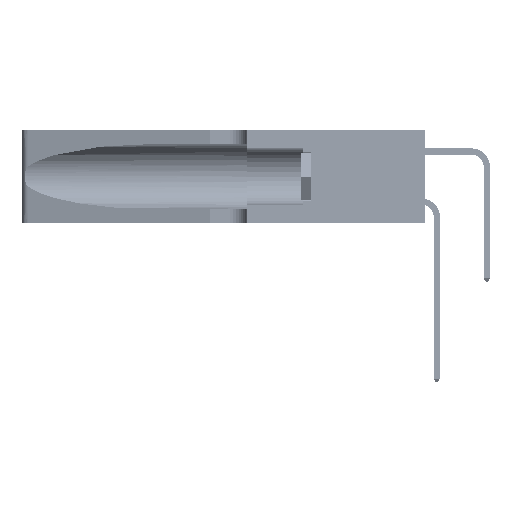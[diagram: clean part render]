
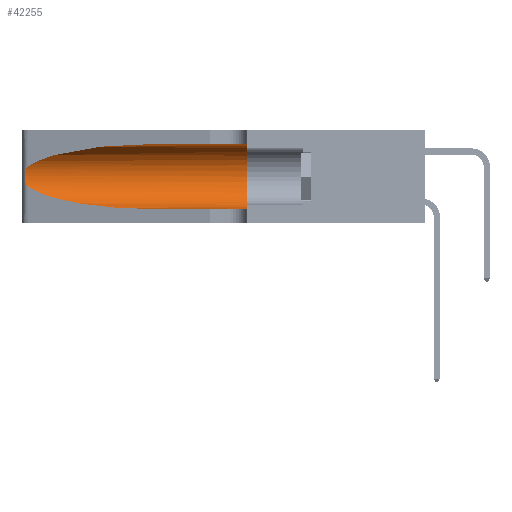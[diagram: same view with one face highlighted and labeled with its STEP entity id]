
A CAD part, left-side view. The second image highlights one B-rep face of the part: STEP entity #42255.
In plain terms, the highlighted cylindrical face has radius 3.308 mm (diameter 6.617 mm), a partial arc.
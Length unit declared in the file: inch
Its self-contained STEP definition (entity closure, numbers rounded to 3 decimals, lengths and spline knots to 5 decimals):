
#624 = VECTOR ( 'NONE', #36243, 39.37008 ) ;
#785 = VERTEX_POINT ( 'NONE', #15672 ) ;
#1450 = CARTESIAN_POINT ( 'NONE',  ( 0.1305, 0.35, 0.05475 ) ) ;
#1660 = ORIENTED_EDGE ( 'NONE', *, *, #38935, .F. ) ;
#1837 = LINE ( 'NONE', #47042, #624 ) ;
#1852 = VERTEX_POINT ( 'NONE', #19064 ) ;
#2015 = CARTESIAN_POINT ( 'NONE',  ( 0.25555, 1.22994, 0.2215 ) ) ;
#2172 = CARTESIAN_POINT ( 'NONE',  ( 0.26018, 1.23835, 0.19895 ) ) ;
#2645 = CIRCLE ( 'NONE', #7533, 0.13025 ) ;
#3365 = VECTOR ( 'NONE', #14960, 39.37008 ) ;
#3502 = EDGE_CURVE ( 'NONE', #17841, #41632, #1837, .T. ) ;
#3715 = CARTESIAN_POINT ( 'NONE',  ( 0.1305, 0.72297, 0.05475 ) ) ;
#5640 = CARTESIAN_POINT ( 'NONE',  ( 0.1305, 0.35, 0.185 ) ) ;
#5896 = CARTESIAN_POINT ( 'NONE',  ( 0.26075, 1.23896, 0.178 ) ) ;
#6258 = EDGE_CURVE ( 'NONE', #11419, #1852, #12007, .T. ) ;
#6636 =( BOUNDED_CURVE ( )  B_SPLINE_CURVE ( 3, ( #35171, #35021, #38819, #17061 ),
 .UNSPECIFIED., .F., .F. ) 
 B_SPLINE_CURVE_WITH_KNOTS ( ( 4, 4 ),
 ( 1.5708, 2.84003 ),
 .UNSPECIFIED. ) 
 CURVE ( )  GEOMETRIC_REPRESENTATION_ITEM ( )  RATIONAL_B_SPLINE_CURVE ( ( 1., 0.87, 0.87, 1. ) ) 
 REPRESENTATION_ITEM ( '' )  );
#6825 = ORIENTED_EDGE ( 'NONE', *, *, #6258, .F. ) ;
#7533 = AXIS2_PLACEMENT_3D ( 'NONE', #5640, #31201, #9362 ) ;
#7587 = CARTESIAN_POINT ( 'NONE',  ( 0.1305, 1.61858, 0.31525 ) ) ;
#8375 = DIRECTION ( 'NONE',  ( 0., 0., -1. ) ) ;
#9362 = DIRECTION ( 'NONE',  ( 0., 0., 1. ) ) ;
#9611 = CARTESIAN_POINT ( 'NONE',  ( 0.25856, 1.23593, 0.16098 ) ) ;
#10188 =( BOUNDED_CURVE ( )  B_SPLINE_CURVE ( 3, ( #18359, #36471, #25668, #3715 ),
 .UNSPECIFIED., .F., .T. ) 
 B_SPLINE_CURVE_WITH_KNOTS ( ( 4, 4 ),
 ( 3.44316, 4.71239 ),
 .UNSPECIFIED. ) 
 CURVE ( )  GEOMETRIC_REPRESENTATION_ITEM ( )  RATIONAL_B_SPLINE_CURVE ( ( 1., 0.87, 0.87, 1. ) ) 
 REPRESENTATION_ITEM ( '' )  );
#11419 = VERTEX_POINT ( 'NONE', #17597 ) ;
#11868 = CARTESIAN_POINT ( 'NONE',  ( 0.1305, 1.61858, 0.185 ) ) ;
#12007 = LINE ( 'NONE', #7587, #3365 ) ;
#13119 = CARTESIAN_POINT ( 'NONE',  ( 0.25487, 1.22718, 0.22369 ) ) ;
#13284 = CARTESIAN_POINT ( 'NONE',  ( 0.25639, 1.23186, 0.15144 ) ) ;
#14960 = DIRECTION ( 'NONE',  ( 0., -1., 0. ) ) ;
#15672 = CARTESIAN_POINT ( 'NONE',  ( 0.25487, 1.22718, 0.14631 ) ) ;
#16975 = CARTESIAN_POINT ( 'NONE',  ( 0.25487, 1.22718, 0.14631 ) ) ;
#17061 = CARTESIAN_POINT ( 'NONE',  ( 0.25487, 1.22718, 0.22369 ) ) ;
#17102 = ORIENTED_EDGE ( 'NONE', *, *, #26921, .T. ) ;
#17597 = CARTESIAN_POINT ( 'NONE',  ( 0.1305, 0.72297, 0.31525 ) ) ;
#17841 = VERTEX_POINT ( 'NONE', #35117 ) ;
#18359 = CARTESIAN_POINT ( 'NONE',  ( 0.25487, 1.22718, 0.14631 ) ) ;
#18668 = B_SPLINE_CURVE_WITH_KNOTS ( 'NONE', 3,
 ( #13119, #2015, #20495, #45914, #24127, #2172, #27794, #5896, #31438, #9611, #35088, #13284, #38726, #16975 ),
 .UNSPECIFIED., .F., .F.,
 ( 4, 2, 2, 2, 2, 2, 4 ),
 ( 0., 0.00027, 0.00053, 0.00107, 0.0016, 0.00187, 0.00214 ),
 .UNSPECIFIED. ) ;
#19064 = CARTESIAN_POINT ( 'NONE',  ( 0.1305, 0.35, 0.31525 ) ) ;
#20077 = ORIENTED_EDGE ( 'NONE', *, *, #41803, .T. ) ;
#20495 = CARTESIAN_POINT ( 'NONE',  ( 0.25639, 1.23184, 0.21858 ) ) ;
#21907 = EDGE_CURVE ( 'NONE', #45333, #785, #18668, .T. ) ;
#24127 = CARTESIAN_POINT ( 'NONE',  ( 0.25854, 1.2359, 0.20912 ) ) ;
#24492 = AXIS2_PLACEMENT_3D ( 'NONE', #11868, #30219, #8375 ) ;
#25386 = ORIENTED_EDGE ( 'NONE', *, *, #3502, .T. ) ;
#25668 = CARTESIAN_POINT ( 'NONE',  ( 0.18966, 0.96281, 0.05475 ) ) ;
#26921 = EDGE_CURVE ( 'NONE', #785, #17841, #10188, .T. ) ;
#27794 = CARTESIAN_POINT ( 'NONE',  ( 0.26075, 1.23896, 0.19203 ) ) ;
#29712 = ORIENTED_EDGE ( 'NONE', *, *, #21907, .T. ) ;
#30219 = DIRECTION ( 'NONE',  ( 0., -1., 0. ) ) ;
#30465 = EDGE_LOOP ( 'NONE', ( #20077, #29712, #17102, #25386, #1660, #6825 ) ) ;
#31201 = DIRECTION ( 'NONE',  ( 0., 1., 0. ) ) ;
#31438 = CARTESIAN_POINT ( 'NONE',  ( 0.26017, 1.23833, 0.17102 ) ) ;
#35021 = CARTESIAN_POINT ( 'NONE',  ( 0.18966, 0.96281, 0.31525 ) ) ;
#35088 = CARTESIAN_POINT ( 'NONE',  ( 0.25789, 1.23486, 0.15765 ) ) ;
#35117 = CARTESIAN_POINT ( 'NONE',  ( 0.1305, 0.72297, 0.05475 ) ) ;
#35139 = FACE_OUTER_BOUND ( 'NONE', #30465, .T. ) ;
#35171 = CARTESIAN_POINT ( 'NONE',  ( 0.1305, 0.72297, 0.31525 ) ) ;
#36243 = DIRECTION ( 'NONE',  ( 0., -1., 0. ) ) ;
#36471 = CARTESIAN_POINT ( 'NONE',  ( 0.2373, 1.15595, 0.08982 ) ) ;
#38726 = CARTESIAN_POINT ( 'NONE',  ( 0.25555, 1.22993, 0.14849 ) ) ;
#38819 = CARTESIAN_POINT ( 'NONE',  ( 0.2373, 1.15595, 0.28018 ) ) ;
#38935 = EDGE_CURVE ( 'NONE', #1852, #41632, #2645, .T. ) ;
#39887 = CARTESIAN_POINT ( 'NONE',  ( 0.25487, 1.22718, 0.22369 ) ) ;
#41632 = VERTEX_POINT ( 'NONE', #1450 ) ;
#41803 = EDGE_CURVE ( 'NONE', #11419, #45333, #6636, .T. ) ;
#42255 = ADVANCED_FACE ( 'NONE', ( #35139 ), #43661, .F. ) ;
#43661 = CYLINDRICAL_SURFACE ( 'NONE', #24492, 0.13025 ) ;
#45333 = VERTEX_POINT ( 'NONE', #39887 ) ;
#45914 = CARTESIAN_POINT ( 'NONE',  ( 0.25787, 1.23484, 0.2124 ) ) ;
#47042 = CARTESIAN_POINT ( 'NONE',  ( 0.1305, 1.61858, 0.05475 ) ) ;
